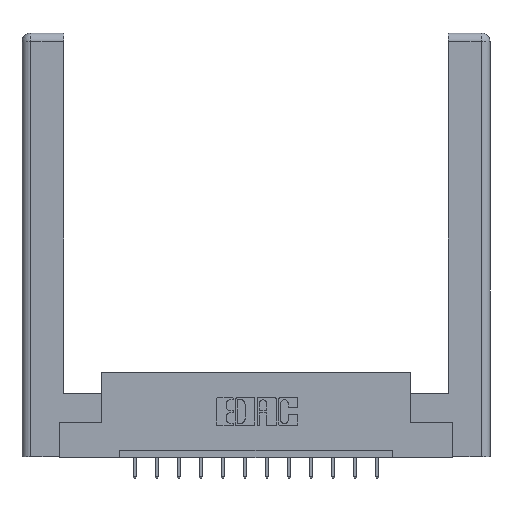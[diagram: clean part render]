
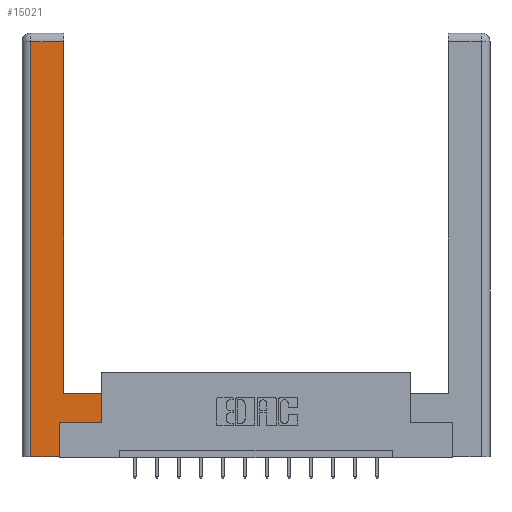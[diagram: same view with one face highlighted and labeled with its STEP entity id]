
A CAD part, top view. The second image highlights one B-rep face of the part: STEP entity #15021.
In plain terms, the highlighted planar face has unit normal (0, 0, 1).
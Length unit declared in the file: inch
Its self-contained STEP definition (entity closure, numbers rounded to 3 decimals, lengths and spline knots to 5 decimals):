
#56 = EDGE_CURVE ( 'NONE', #1115, #10328, #14541, .T. ) ;
#112 = VECTOR ( 'NONE', #6096, 39.37008 ) ;
#698 = DIRECTION ( 'NONE',  ( -1., 0., 0. ) ) ;
#706 = VECTOR ( 'NONE', #14371, 39.37008 ) ;
#927 = ORIENTED_EDGE ( 'NONE', *, *, #8915, .T. ) ;
#1115 = VERTEX_POINT ( 'NONE', #12542 ) ;
#1353 = DIRECTION ( 'NONE',  ( -1., 0., 0. ) ) ;
#1535 = EDGE_CURVE ( 'NONE', #10328, #11078, #3051, .T. ) ;
#2642 = ORIENTED_EDGE ( 'NONE', *, *, #11870, .T. ) ;
#2766 = CARTESIAN_POINT ( 'NONE',  ( 0.265, 0., 0. ) ) ;
#3049 = VERTEX_POINT ( 'NONE', #4362 ) ;
#3051 = LINE ( 'NONE', #3849, #11053 ) ;
#3096 = FACE_OUTER_BOUND ( 'NONE', #4413, .T. ) ;
#3302 = LINE ( 'NONE', #14177, #11316 ) ;
#3400 = CARTESIAN_POINT ( 'NONE',  ( 0.565, 0.245, 0. ) ) ;
#3849 = CARTESIAN_POINT ( 'NONE',  ( 0.0615, 0., 0. ) ) ;
#4362 = CARTESIAN_POINT ( 'NONE',  ( 0.265, 0.245, 0. ) ) ;
#4369 = CARTESIAN_POINT ( 'NONE',  ( 0.0615, 0., 0. ) ) ;
#4413 = EDGE_LOOP ( 'NONE', ( #10884, #7661, #9343, #2642, #927, #7121, #6836, #15068 ) ) ;
#4509 = CARTESIAN_POINT ( 'NONE',  ( 0.265, 0.245, 0. ) ) ;
#4694 = CARTESIAN_POINT ( 'NONE',  ( 0.565, 0.245, 0. ) ) ;
#5212 = AXIS2_PLACEMENT_3D ( 'NONE', #14132, #7291, #11183 ) ;
#5217 = EDGE_CURVE ( 'NONE', #3049, #9579, #13182, .T. ) ;
#5664 = LINE ( 'NONE', #14713, #8490 ) ;
#6033 = EDGE_CURVE ( 'NONE', #9579, #10511, #5664, .T. ) ;
#6096 = DIRECTION ( 'NONE',  ( 1., 0., 0. ) ) ;
#6836 = ORIENTED_EDGE ( 'NONE', *, *, #6033, .T. ) ;
#6931 = DIRECTION ( 'NONE',  ( 0., 1., 0. ) ) ;
#7121 = ORIENTED_EDGE ( 'NONE', *, *, #5217, .T. ) ;
#7291 = DIRECTION ( 'NONE',  ( 0., 0., -1. ) ) ;
#7526 = CARTESIAN_POINT ( 'NONE',  ( 0.295, 0.45, 0. ) ) ;
#7661 = ORIENTED_EDGE ( 'NONE', *, *, #56, .T. ) ;
#7854 = CARTESIAN_POINT ( 'NONE',  ( 0.0615, 2.94, 0. ) ) ;
#7911 = LINE ( 'NONE', #4509, #10518 ) ;
#8006 = LINE ( 'NONE', #14319, #706 ) ;
#8490 = VECTOR ( 'NONE', #9784, 39.37008 ) ;
#8550 = PLANE ( 'NONE',  #5212 ) ;
#8715 = VERTEX_POINT ( 'NONE', #12122 ) ;
#8763 = DIRECTION ( 'NONE',  ( 0., -1., 0. ) ) ;
#8915 = EDGE_CURVE ( 'NONE', #13904, #3049, #7911, .T. ) ;
#9343 = ORIENTED_EDGE ( 'NONE', *, *, #1535, .T. ) ;
#9579 = VERTEX_POINT ( 'NONE', #3400 ) ;
#9784 = DIRECTION ( 'NONE',  ( 0., 1., 0. ) ) ;
#10328 = VERTEX_POINT ( 'NONE', #12472 ) ;
#10511 = VERTEX_POINT ( 'NONE', #11679 ) ;
#10518 = VECTOR ( 'NONE', #6931, 39.37008 ) ;
#10884 = ORIENTED_EDGE ( 'NONE', *, *, #14035, .T. ) ;
#11053 = VECTOR ( 'NONE', #8763, 39.37008 ) ;
#11078 = VERTEX_POINT ( 'NONE', #4369 ) ;
#11183 = DIRECTION ( 'NONE',  ( -1., 0., 0. ) ) ;
#11316 = VECTOR ( 'NONE', #12886, 39.37008 ) ;
#11679 = CARTESIAN_POINT ( 'NONE',  ( 0.565, 0.45, 0. ) ) ;
#11870 = EDGE_CURVE ( 'NONE', #11078, #13904, #8006, .T. ) ;
#11903 = LINE ( 'NONE', #7526, #14126 ) ;
#12122 = CARTESIAN_POINT ( 'NONE',  ( 0.295, 0.45, 0. ) ) ;
#12472 = CARTESIAN_POINT ( 'NONE',  ( 0.0615, 2.94, 0. ) ) ;
#12542 = CARTESIAN_POINT ( 'NONE',  ( 0.295, 2.94, 0. ) ) ;
#12881 = EDGE_CURVE ( 'NONE', #10511, #8715, #11903, .T. ) ;
#12886 = DIRECTION ( 'NONE',  ( 0., 1., 0. ) ) ;
#13182 = LINE ( 'NONE', #4694, #112 ) ;
#13416 = VECTOR ( 'NONE', #698, 39.37008 ) ;
#13904 = VERTEX_POINT ( 'NONE', #2766 ) ;
#14035 = EDGE_CURVE ( 'NONE', #8715, #1115, #3302, .T. ) ;
#14126 = VECTOR ( 'NONE', #1353, 39.37008 ) ;
#14132 = CARTESIAN_POINT ( 'NONE',  ( 0., 0., 0. ) ) ;
#14177 = CARTESIAN_POINT ( 'NONE',  ( 0.295, 3., 0. ) ) ;
#14319 = CARTESIAN_POINT ( 'NONE',  ( 0.265, 0., 0. ) ) ;
#14371 = DIRECTION ( 'NONE',  ( 1., 0., 0. ) ) ;
#14541 = LINE ( 'NONE', #7854, #13416 ) ;
#14713 = CARTESIAN_POINT ( 'NONE',  ( 0.565, 0.45, 0. ) ) ;
#15021 = ADVANCED_FACE ( 'NONE', ( #3096 ), #8550, .F. ) ;
#15068 = ORIENTED_EDGE ( 'NONE', *, *, #12881, .T. ) ;
